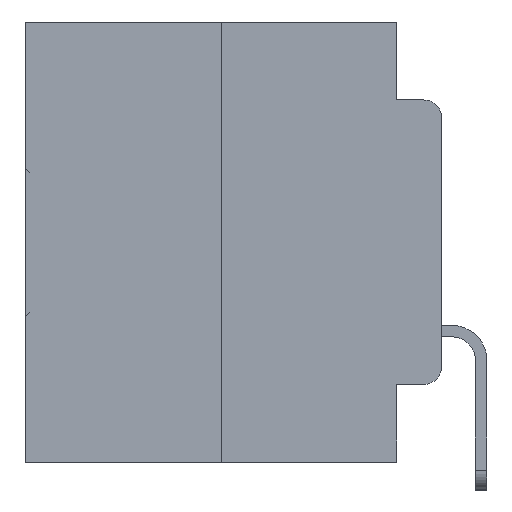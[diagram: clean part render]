
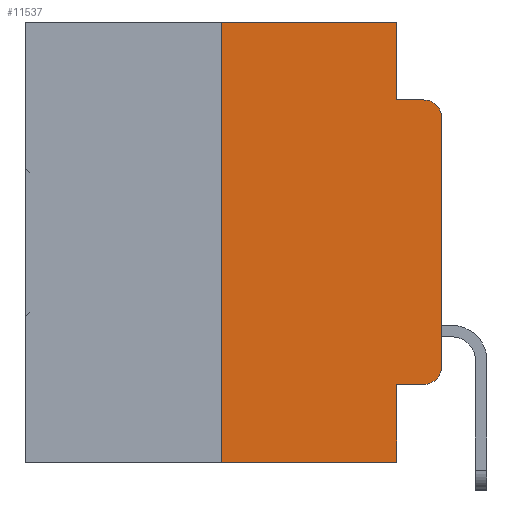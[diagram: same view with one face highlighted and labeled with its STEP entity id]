
A CAD part, left-side view. The second image highlights one B-rep face of the part: STEP entity #11537.
In plain terms, the highlighted planar face has unit normal (-1, 0, 0).
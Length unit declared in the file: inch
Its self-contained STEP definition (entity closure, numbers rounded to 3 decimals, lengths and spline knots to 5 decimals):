
#25 = CARTESIAN_POINT ( 'NONE',  ( 0., 0.051, -0.5 ) ) ;
#100 = EDGE_CURVE ( 'NONE', #28448, #1120, #6526, .T. ) ;
#1120 = VERTEX_POINT ( 'NONE', #30748 ) ;
#1267 = EDGE_LOOP ( 'NONE', ( #12289, #12189, #8510, #1981, #9018, #16166, #14683, #13410, #12617, #8655 ) ) ;
#1311 = CIRCLE ( 'NONE', #10646, 0.02 ) ;
#1709 = EDGE_CURVE ( 'NONE', #10340, #2599, #2810, .T. ) ;
#1981 = ORIENTED_EDGE ( 'NONE', *, *, #100, .F. ) ;
#1999 = CARTESIAN_POINT ( 'NONE',  ( 0., 0.473, 0. ) ) ;
#2599 = VERTEX_POINT ( 'NONE', #25 ) ;
#2810 = LINE ( 'NONE', #12048, #9785 ) ;
#2830 = EDGE_CURVE ( 'NONE', #10340, #6152, #30523, .T. ) ;
#3001 = CARTESIAN_POINT ( 'NONE',  ( 0., 0., -0.1085 ) ) ;
#3219 = CARTESIAN_POINT ( 'NONE',  ( 0., 0.02, -0.3915 ) ) ;
#3402 = DIRECTION ( 'NONE',  ( 0., -1., 0. ) ) ;
#3670 = CARTESIAN_POINT ( 'NONE',  ( 0., 0.051, -0.4115 ) ) ;
#4108 = EDGE_CURVE ( 'NONE', #19829, #11304, #21987, .T. ) ;
#4154 = CARTESIAN_POINT ( 'NONE',  ( 0., 0., 0. ) ) ;
#4653 = DIRECTION ( 'NONE',  ( 0., 0., 1. ) ) ;
#4783 = EDGE_CURVE ( 'NONE', #29764, #27826, #20037, .T. ) ;
#4984 = CIRCLE ( 'NONE', #21430, 0.02 ) ;
#5147 = VECTOR ( 'NONE', #16471, 39.37008 ) ;
#5185 = EDGE_CURVE ( 'NONE', #11304, #16419, #1311, .T. ) ;
#5196 = VECTOR ( 'NONE', #14950, 39.37008 ) ;
#5842 = DIRECTION ( 'NONE',  ( 0., 0., -1. ) ) ;
#6152 = VERTEX_POINT ( 'NONE', #14755 ) ;
#6526 = LINE ( 'NONE', #29638, #19897 ) ;
#8333 = EDGE_CURVE ( 'NONE', #6152, #19829, #4984, .T. ) ;
#8510 = ORIENTED_EDGE ( 'NONE', *, *, #20794, .F. ) ;
#8655 = ORIENTED_EDGE ( 'NONE', *, *, #8333, .T. ) ;
#8796 = VECTOR ( 'NONE', #16930, 39.37008 ) ;
#9018 = ORIENTED_EDGE ( 'NONE', *, *, #13617, .F. ) ;
#9167 = PLANE ( 'NONE',  #29443 ) ;
#9785 = VECTOR ( 'NONE', #28756, 39.37008 ) ;
#9903 = CARTESIAN_POINT ( 'NONE',  ( 0., 0.02, -0.0885 ) ) ;
#10340 = VERTEX_POINT ( 'NONE', #16791 ) ;
#10646 = AXIS2_PLACEMENT_3D ( 'NONE', #28822, #14485, #31178 ) ;
#11009 = VECTOR ( 'NONE', #3402, 39.37008 ) ;
#11304 = VERTEX_POINT ( 'NONE', #3001 ) ;
#11537 = ADVANCED_FACE ( 'NONE', ( #18622 ), #9167, .F. ) ;
#11794 = DIRECTION ( 'NONE',  ( 1., 0., 0. ) ) ;
#12048 = CARTESIAN_POINT ( 'NONE',  ( 0., 0.051, 0. ) ) ;
#12189 = ORIENTED_EDGE ( 'NONE', *, *, #5185, .T. ) ;
#12289 = ORIENTED_EDGE ( 'NONE', *, *, #4108, .T. ) ;
#12617 = ORIENTED_EDGE ( 'NONE', *, *, #2830, .T. ) ;
#12863 = DIRECTION ( 'NONE',  ( 0., 0., -1. ) ) ;
#13410 = ORIENTED_EDGE ( 'NONE', *, *, #1709, .F. ) ;
#13613 = VECTOR ( 'NONE', #4653, 39.37008 ) ;
#13617 = EDGE_CURVE ( 'NONE', #27826, #28448, #25777, .T. ) ;
#14485 = DIRECTION ( 'NONE',  ( -1., 0., 0. ) ) ;
#14577 = CARTESIAN_POINT ( 'NONE',  ( 0., 0.051, 0. ) ) ;
#14683 = ORIENTED_EDGE ( 'NONE', *, *, #23547, .T. ) ;
#14755 = CARTESIAN_POINT ( 'NONE',  ( 0., 0.02, -0.4115 ) ) ;
#14950 = DIRECTION ( 'NONE',  ( 0., -1., 0. ) ) ;
#15525 = CARTESIAN_POINT ( 'NONE',  ( 0., 0.25, 0. ) ) ;
#16116 = LINE ( 'NONE', #31853, #28048 ) ;
#16166 = ORIENTED_EDGE ( 'NONE', *, *, #4783, .F. ) ;
#16419 = VERTEX_POINT ( 'NONE', #9903 ) ;
#16471 = DIRECTION ( 'NONE',  ( 0., -1., 0. ) ) ;
#16791 = CARTESIAN_POINT ( 'NONE',  ( 0., 0.051, -0.4115 ) ) ;
#16930 = DIRECTION ( 'NONE',  ( 0., 0., 1. ) ) ;
#16966 = CARTESIAN_POINT ( 'NONE',  ( 0., 0.25, -0.5 ) ) ;
#18622 = FACE_OUTER_BOUND ( 'NONE', #1267, .T. ) ;
#19829 = VERTEX_POINT ( 'NONE', #23254 ) ;
#19897 = VECTOR ( 'NONE', #12863, 39.37008 ) ;
#20036 = DIRECTION ( 'NONE',  ( 0., -1., 0. ) ) ;
#20037 = LINE ( 'NONE', #26896, #13613 ) ;
#20794 = EDGE_CURVE ( 'NONE', #1120, #16419, #30266, .T. ) ;
#20865 = DIRECTION ( 'NONE',  ( -1., 0., 0. ) ) ;
#21430 = AXIS2_PLACEMENT_3D ( 'NONE', #3219, #20865, #5842 ) ;
#21515 = CARTESIAN_POINT ( 'NONE',  ( 0., 0.473, 0. ) ) ;
#21987 = LINE ( 'NONE', #4154, #8796 ) ;
#23254 = CARTESIAN_POINT ( 'NONE',  ( 0., 0., -0.3915 ) ) ;
#23547 = EDGE_CURVE ( 'NONE', #29764, #2599, #16116, .T. ) ;
#24237 = CARTESIAN_POINT ( 'NONE',  ( 0., 0.051, -0.0885 ) ) ;
#25777 = LINE ( 'NONE', #1999, #5196 ) ;
#26896 = CARTESIAN_POINT ( 'NONE',  ( 0., 0.25, 0. ) ) ;
#27826 = VERTEX_POINT ( 'NONE', #15525 ) ;
#28048 = VECTOR ( 'NONE', #20036, 39.37008 ) ;
#28448 = VERTEX_POINT ( 'NONE', #14577 ) ;
#28667 = DIRECTION ( 'NONE',  ( 0., 0., -1. ) ) ;
#28756 = DIRECTION ( 'NONE',  ( 0., 0., -1. ) ) ;
#28822 = CARTESIAN_POINT ( 'NONE',  ( 0., 0.02, -0.1085 ) ) ;
#29443 = AXIS2_PLACEMENT_3D ( 'NONE', #21515, #11794, #28667 ) ;
#29638 = CARTESIAN_POINT ( 'NONE',  ( 0., 0.051, 0. ) ) ;
#29764 = VERTEX_POINT ( 'NONE', #16966 ) ;
#30266 = LINE ( 'NONE', #24237, #11009 ) ;
#30523 = LINE ( 'NONE', #3670, #5147 ) ;
#30748 = CARTESIAN_POINT ( 'NONE',  ( 0., 0.051, -0.0885 ) ) ;
#31178 = DIRECTION ( 'NONE',  ( 0., 0., -1. ) ) ;
#31853 = CARTESIAN_POINT ( 'NONE',  ( 0., 0.473, -0.5 ) ) ;
